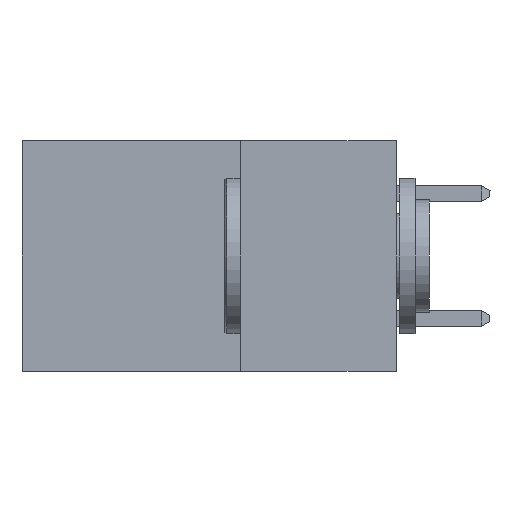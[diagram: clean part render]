
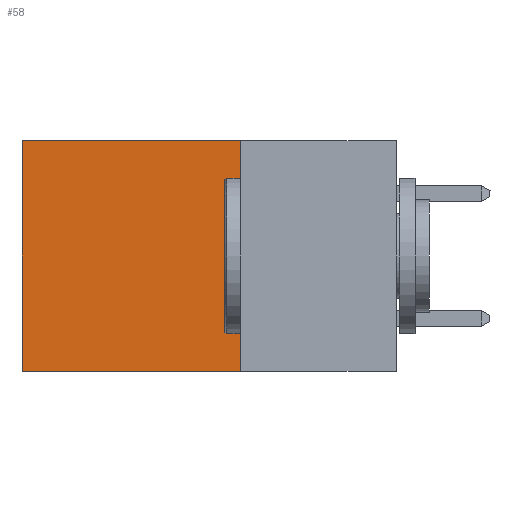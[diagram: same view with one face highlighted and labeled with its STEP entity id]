
A CAD part, left-side view. The second image highlights one B-rep face of the part: STEP entity #58.
In plain terms, the highlighted planar face has unit normal (-1, 0, 0).
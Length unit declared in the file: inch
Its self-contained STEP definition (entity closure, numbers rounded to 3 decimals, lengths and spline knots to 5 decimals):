
#58 = ADVANCED_FACE ( 'NONE', ( #10946 ), #12151, .F. ) ;
#994 = LINE ( 'NONE', #10657, #9284 ) ;
#1889 = CARTESIAN_POINT ( 'NONE',  ( 0.298, 0.25, -0.37 ) ) ;
#2032 = CARTESIAN_POINT ( 'NONE',  ( 0.298, 0.6, 0. ) ) ;
#2527 = EDGE_CURVE ( 'NONE', #6114, #11685, #4626, .T. ) ;
#2673 = DIRECTION ( 'NONE',  ( 0., 1., 0. ) ) ;
#2973 = DIRECTION ( 'NONE',  ( 1., 0., 0. ) ) ;
#3436 = CARTESIAN_POINT ( 'NONE',  ( 0.298, 0.25, 0. ) ) ;
#3896 = VECTOR ( 'NONE', #6532, 39.37008 ) ;
#4181 = VERTEX_POINT ( 'NONE', #9082 ) ;
#4468 = EDGE_CURVE ( 'NONE', #11044, #6114, #994, .T. ) ;
#4626 = LINE ( 'NONE', #1889, #10134 ) ;
#5104 = ORIENTED_EDGE ( 'NONE', *, *, #4468, .F. ) ;
#5394 = CARTESIAN_POINT ( 'NONE',  ( 0.298, 0.25, 0. ) ) ;
#5627 = EDGE_CURVE ( 'NONE', #4181, #11685, #6846, .T. ) ;
#5747 = DIRECTION ( 'NONE',  ( 0., 0., -1. ) ) ;
#5771 = VECTOR ( 'NONE', #5747, 39.37008 ) ;
#6114 = VERTEX_POINT ( 'NONE', #13682 ) ;
#6532 = DIRECTION ( 'NONE',  ( 0., 1., 0. ) ) ;
#6662 = AXIS2_PLACEMENT_3D ( 'NONE', #12318, #2973, #12642 ) ;
#6846 = LINE ( 'NONE', #2032, #5771 ) ;
#6892 = LINE ( 'NONE', #5394, #3896 ) ;
#7064 = EDGE_CURVE ( 'NONE', #11044, #4181, #6892, .T. ) ;
#8230 = ORIENTED_EDGE ( 'NONE', *, *, #5627, .T. ) ;
#8785 = ORIENTED_EDGE ( 'NONE', *, *, #7064, .T. ) ;
#9082 = CARTESIAN_POINT ( 'NONE',  ( 0.298, 0.6, 0. ) ) ;
#9284 = VECTOR ( 'NONE', #10553, 39.37008 ) ;
#10014 = CARTESIAN_POINT ( 'NONE',  ( 0.298, 0.6, -0.37 ) ) ;
#10134 = VECTOR ( 'NONE', #2673, 39.37008 ) ;
#10522 = EDGE_LOOP ( 'NONE', ( #8230, #13711, #5104, #8785 ) ) ;
#10553 = DIRECTION ( 'NONE',  ( 0., 0., -1. ) ) ;
#10657 = CARTESIAN_POINT ( 'NONE',  ( 0.298, 0.25, 0. ) ) ;
#10946 = FACE_OUTER_BOUND ( 'NONE', #10522, .T. ) ;
#11044 = VERTEX_POINT ( 'NONE', #3436 ) ;
#11685 = VERTEX_POINT ( 'NONE', #10014 ) ;
#12151 = PLANE ( 'NONE',  #6662 ) ;
#12318 = CARTESIAN_POINT ( 'NONE',  ( 0.298, 0.25, 0. ) ) ;
#12642 = DIRECTION ( 'NONE',  ( 0., 0., -1. ) ) ;
#13682 = CARTESIAN_POINT ( 'NONE',  ( 0.298, 0.25, -0.37 ) ) ;
#13711 = ORIENTED_EDGE ( 'NONE', *, *, #2527, .F. ) ;
